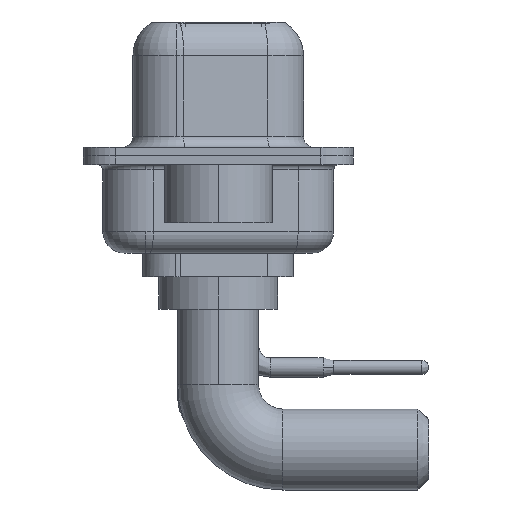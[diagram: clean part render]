
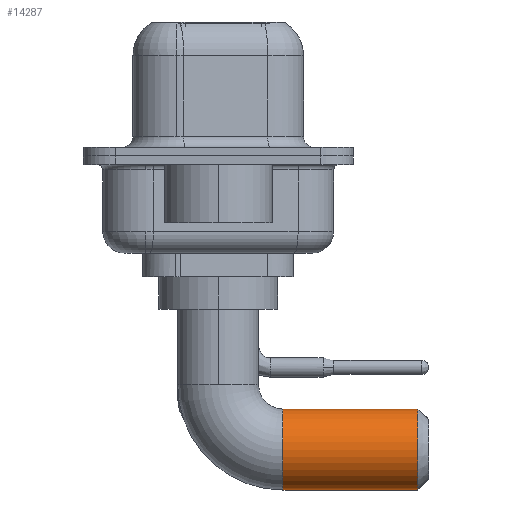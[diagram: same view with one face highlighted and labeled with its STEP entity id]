
A CAD part, left-side view. The second image highlights one B-rep face of the part: STEP entity #14287.
In plain terms, the highlighted cylindrical face has radius 1.875 mm (diameter 3.75 mm), a partial arc.
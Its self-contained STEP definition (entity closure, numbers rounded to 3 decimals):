
#613 = ORIENTED_EDGE ( 'NONE', *, *, #3389, .T. ) ;
#1636 = DIRECTION ( 'NONE',  ( 0., 1., 0. ) ) ;
#1711 = AXIS2_PLACEMENT_3D ( 'NONE', #9862, #12616, #16296 ) ;
#1808 = VERTEX_POINT ( 'NONE', #8685 ) ;
#1911 = VERTEX_POINT ( 'NONE', #17001 ) ;
#1935 = LINE ( 'NONE', #12886, #13978 ) ;
#2034 = CIRCLE ( 'NONE', #3047, 1.875 ) ;
#2096 = VERTEX_POINT ( 'NONE', #17210 ) ;
#2150 = DIRECTION ( 'NONE',  ( -1., 0., 0. ) ) ;
#2446 = ORIENTED_EDGE ( 'NONE', *, *, #12586, .T. ) ;
#2665 = CARTESIAN_POINT ( 'NONE',  ( 0., -9.25, -8.375 ) ) ;
#3047 = AXIS2_PLACEMENT_3D ( 'NONE', #13091, #3826, #2150 ) ;
#3389 = EDGE_CURVE ( 'NONE', #1911, #12875, #1935, .T. ) ;
#3507 = DIRECTION ( 'NONE',  ( 0., -1., 0. ) ) ;
#3826 = DIRECTION ( 'NONE',  ( 0., -1., 0. ) ) ;
#5369 = CIRCLE ( 'NONE', #18171, 1.875 ) ;
#6322 = EDGE_LOOP ( 'NONE', ( #11951, #8025, #613, #2446 ) ) ;
#6359 = CARTESIAN_POINT ( 'NONE',  ( 0., -9.25, -6.5 ) ) ;
#6980 = VECTOR ( 'NONE', #8277, 1000. ) ;
#7883 = FACE_OUTER_BOUND ( 'NONE', #6322, .T. ) ;
#8025 = ORIENTED_EDGE ( 'NONE', *, *, #12610, .T. ) ;
#8063 = DIRECTION ( 'NONE',  ( 0., 0., -1. ) ) ;
#8277 = DIRECTION ( 'NONE',  ( 0., -1., 0. ) ) ;
#8685 = CARTESIAN_POINT ( 'NONE',  ( 0., -9.25, -4.625 ) ) ;
#9862 = CARTESIAN_POINT ( 'NONE',  ( 0., -3., -6.5 ) ) ;
#10103 = EDGE_CURVE ( 'NONE', #2096, #1808, #20506, .T. ) ;
#11951 = ORIENTED_EDGE ( 'NONE', *, *, #10103, .F. ) ;
#12586 = EDGE_CURVE ( 'NONE', #12875, #1808, #5369, .T. ) ;
#12610 = EDGE_CURVE ( 'NONE', #2096, #1911, #2034, .T. ) ;
#12616 = DIRECTION ( 'NONE',  ( 0., -1., 0. ) ) ;
#12713 = CYLINDRICAL_SURFACE ( 'NONE', #1711, 1.875 ) ;
#12875 = VERTEX_POINT ( 'NONE', #2665 ) ;
#12886 = CARTESIAN_POINT ( 'NONE',  ( 0., -3., -8.375 ) ) ;
#13091 = CARTESIAN_POINT ( 'NONE',  ( 0., -3., -6.5 ) ) ;
#13978 = VECTOR ( 'NONE', #3507, 1000. ) ;
#14287 = ADVANCED_FACE ( 'NONE', ( #7883 ), #12713, .T. ) ;
#16296 = DIRECTION ( 'NONE',  ( 0., 0., -1. ) ) ;
#16381 = CARTESIAN_POINT ( 'NONE',  ( 0., -3., -4.625 ) ) ;
#17001 = CARTESIAN_POINT ( 'NONE',  ( 0., -3., -8.375 ) ) ;
#17210 = CARTESIAN_POINT ( 'NONE',  ( 0., -3., -4.625 ) ) ;
#18171 = AXIS2_PLACEMENT_3D ( 'NONE', #6359, #1636, #8063 ) ;
#20506 = LINE ( 'NONE', #16381, #6980 ) ;
